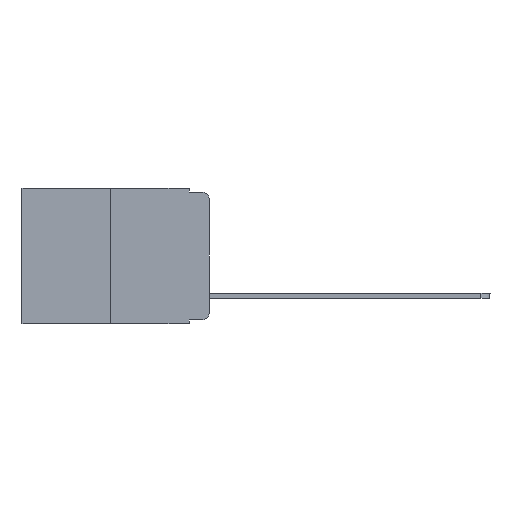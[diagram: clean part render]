
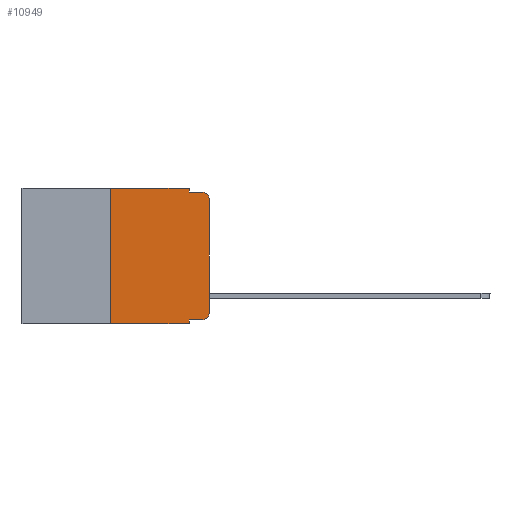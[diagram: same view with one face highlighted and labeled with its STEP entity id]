
A CAD part, left-side view. The second image highlights one B-rep face of the part: STEP entity #10949.
In plain terms, the highlighted planar face has unit normal (-1, 0, 0).
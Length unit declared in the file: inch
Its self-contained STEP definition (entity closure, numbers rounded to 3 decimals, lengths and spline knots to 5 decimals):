
#22 = VERTEX_POINT ( 'NONE', #11755 ) ;
#283 = DIRECTION ( 'NONE',  ( 1., 0., 0. ) ) ;
#345 = ORIENTED_EDGE ( 'NONE', *, *, #376, .F. ) ;
#376 = EDGE_CURVE ( 'NONE', #22, #17918, #4168, .T. ) ;
#652 = DIRECTION ( 'NONE',  ( 0., 0., -1. ) ) ;
#700 = CARTESIAN_POINT ( 'NONE',  ( 0., 0.051, -0.01 ) ) ;
#811 = VECTOR ( 'NONE', #5532, 39.37008 ) ;
#963 = VECTOR ( 'NONE', #10236, 39.37008 ) ;
#1301 = CARTESIAN_POINT ( 'NONE',  ( 0., 0.02, -0.01 ) ) ;
#2033 = DIRECTION ( 'NONE',  ( 0., 0., 1. ) ) ;
#2238 = CARTESIAN_POINT ( 'NONE',  ( 0., 0.051, -0.01 ) ) ;
#2551 = EDGE_CURVE ( 'NONE', #15183, #12077, #11512, .T. ) ;
#2613 = CARTESIAN_POINT ( 'NONE',  ( 0., 0.051, 0. ) ) ;
#2631 = CARTESIAN_POINT ( 'NONE',  ( 0., 0.051, 0. ) ) ;
#2729 = AXIS2_PLACEMENT_3D ( 'NONE', #17983, #10366, #9010 ) ;
#2887 = CARTESIAN_POINT ( 'NONE',  ( 0., 0., -0.03 ) ) ;
#2964 = CARTESIAN_POINT ( 'NONE',  ( 0., 0.473, -0.343 ) ) ;
#3192 = EDGE_CURVE ( 'NONE', #11930, #4742, #11156, .T. ) ;
#3547 = DIRECTION ( 'NONE',  ( -1., 0., 0. ) ) ;
#4142 = VECTOR ( 'NONE', #12872, 39.37008 ) ;
#4168 = LINE ( 'NONE', #2613, #811 ) ;
#4354 = CARTESIAN_POINT ( 'NONE',  ( 0., 0.473, 0. ) ) ;
#4388 = EDGE_CURVE ( 'NONE', #9909, #17918, #10219, .T. ) ;
#4543 = PLANE ( 'NONE',  #15069 ) ;
#4742 = VERTEX_POINT ( 'NONE', #1301 ) ;
#5247 = CARTESIAN_POINT ( 'NONE',  ( 0., 0., 0. ) ) ;
#5532 = DIRECTION ( 'NONE',  ( 0., 0., -1. ) ) ;
#5759 = VERTEX_POINT ( 'NONE', #12390 ) ;
#6139 = VECTOR ( 'NONE', #12655, 39.37008 ) ;
#6195 = AXIS2_PLACEMENT_3D ( 'NONE', #15172, #3547, #16694 ) ;
#6372 = DIRECTION ( 'NONE',  ( 0., 0., 1. ) ) ;
#6769 = LINE ( 'NONE', #18535, #6139 ) ;
#7544 = VERTEX_POINT ( 'NONE', #2887 ) ;
#8753 = ORIENTED_EDGE ( 'NONE', *, *, #4388, .T. ) ;
#9010 = DIRECTION ( 'NONE',  ( 0., 0., -1. ) ) ;
#9225 = ORIENTED_EDGE ( 'NONE', *, *, #18544, .T. ) ;
#9727 = CARTESIAN_POINT ( 'NONE',  ( 0., 0.25, -0.343 ) ) ;
#9819 = ORIENTED_EDGE ( 'NONE', *, *, #16899, .T. ) ;
#9850 = EDGE_CURVE ( 'NONE', #12077, #11930, #15357, .T. ) ;
#9909 = VERTEX_POINT ( 'NONE', #9727 ) ;
#10219 = LINE ( 'NONE', #2964, #18522 ) ;
#10236 = DIRECTION ( 'NONE',  ( 0., -1., 0. ) ) ;
#10366 = DIRECTION ( 'NONE',  ( -1., 0., 0. ) ) ;
#10901 = LINE ( 'NONE', #18225, #16973 ) ;
#10949 = ADVANCED_FACE ( 'NONE', ( #17758 ), #4543, .F. ) ;
#11075 = CIRCLE ( 'NONE', #2729, 0.02 ) ;
#11156 = LINE ( 'NONE', #2238, #4142 ) ;
#11512 = LINE ( 'NONE', #4354, #963 ) ;
#11587 = DIRECTION ( 'NONE',  ( 0., -1., 0. ) ) ;
#11755 = CARTESIAN_POINT ( 'NONE',  ( 0., 0.051, -0.333 ) ) ;
#11930 = VERTEX_POINT ( 'NONE', #700 ) ;
#11931 = EDGE_LOOP ( 'NONE', ( #18313, #9819, #16166, #15655, #14770, #14168, #8753, #345, #12676, #9225 ) ) ;
#12077 = VERTEX_POINT ( 'NONE', #2631 ) ;
#12390 = CARTESIAN_POINT ( 'NONE',  ( 0., 0.02, -0.333 ) ) ;
#12574 = LINE ( 'NONE', #5247, #17242 ) ;
#12655 = DIRECTION ( 'NONE',  ( 0., -1., 0. ) ) ;
#12676 = ORIENTED_EDGE ( 'NONE', *, *, #15454, .T. ) ;
#12872 = DIRECTION ( 'NONE',  ( 0., -1., 0. ) ) ;
#13098 = CARTESIAN_POINT ( 'NONE',  ( 0., 0.051, -0.343 ) ) ;
#13146 = VERTEX_POINT ( 'NONE', #15315 ) ;
#13524 = CARTESIAN_POINT ( 'NONE',  ( 0., 0.473, 0. ) ) ;
#13901 = CARTESIAN_POINT ( 'NONE',  ( 0., 0.051, 0. ) ) ;
#14168 = ORIENTED_EDGE ( 'NONE', *, *, #16957, .F. ) ;
#14770 = ORIENTED_EDGE ( 'NONE', *, *, #2551, .F. ) ;
#14803 = DIRECTION ( 'NONE',  ( 0., 0., -1. ) ) ;
#15069 = AXIS2_PLACEMENT_3D ( 'NONE', #13524, #283, #14803 ) ;
#15172 = CARTESIAN_POINT ( 'NONE',  ( 0., 0.02, -0.03 ) ) ;
#15183 = VERTEX_POINT ( 'NONE', #16996 ) ;
#15315 = CARTESIAN_POINT ( 'NONE',  ( 0., 0., -0.313 ) ) ;
#15357 = LINE ( 'NONE', #13901, #16865 ) ;
#15454 = EDGE_CURVE ( 'NONE', #22, #5759, #6769, .T. ) ;
#15655 = ORIENTED_EDGE ( 'NONE', *, *, #9850, .F. ) ;
#16166 = ORIENTED_EDGE ( 'NONE', *, *, #3192, .F. ) ;
#16367 = CIRCLE ( 'NONE', #6195, 0.02 ) ;
#16694 = DIRECTION ( 'NONE',  ( 0., 0., -1. ) ) ;
#16865 = VECTOR ( 'NONE', #652, 39.37008 ) ;
#16899 = EDGE_CURVE ( 'NONE', #7544, #4742, #16367, .T. ) ;
#16957 = EDGE_CURVE ( 'NONE', #9909, #15183, #10901, .T. ) ;
#16973 = VECTOR ( 'NONE', #6372, 39.37008 ) ;
#16996 = CARTESIAN_POINT ( 'NONE',  ( 0., 0.25, 0. ) ) ;
#17242 = VECTOR ( 'NONE', #2033, 39.37008 ) ;
#17758 = FACE_OUTER_BOUND ( 'NONE', #11931, .T. ) ;
#17918 = VERTEX_POINT ( 'NONE', #13098 ) ;
#17983 = CARTESIAN_POINT ( 'NONE',  ( 0., 0.02, -0.313 ) ) ;
#18225 = CARTESIAN_POINT ( 'NONE',  ( 0., 0.25, 0. ) ) ;
#18313 = ORIENTED_EDGE ( 'NONE', *, *, #18712, .T. ) ;
#18522 = VECTOR ( 'NONE', #11587, 39.37008 ) ;
#18535 = CARTESIAN_POINT ( 'NONE',  ( 0., 0.051, -0.333 ) ) ;
#18544 = EDGE_CURVE ( 'NONE', #5759, #13146, #11075, .T. ) ;
#18712 = EDGE_CURVE ( 'NONE', #13146, #7544, #12574, .T. ) ;
